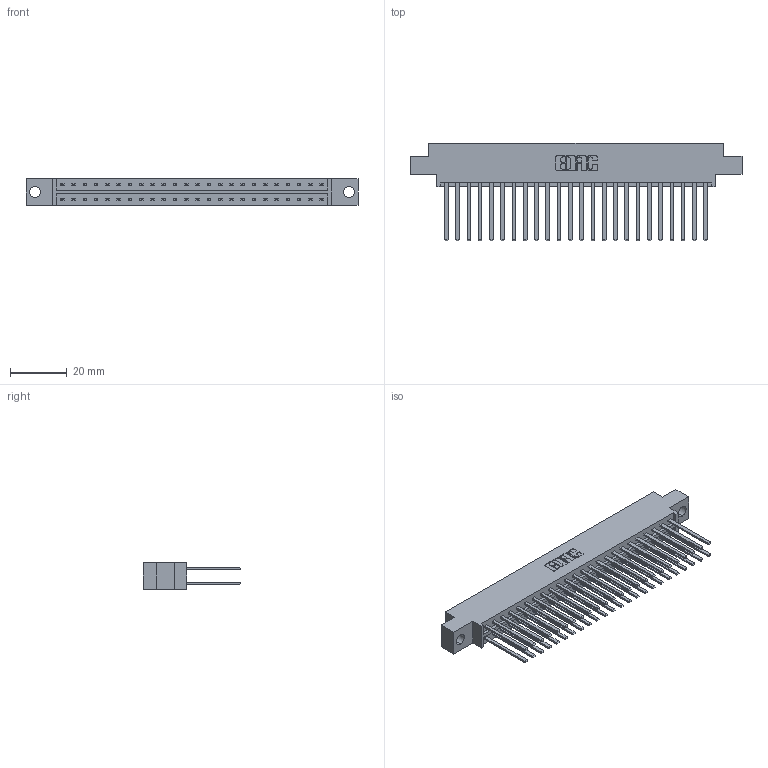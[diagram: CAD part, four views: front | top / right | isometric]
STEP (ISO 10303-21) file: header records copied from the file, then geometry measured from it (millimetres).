
FILE_DESCRIPTION (( 'STEP AP203' ), '1' );
FILE_NAME ('833-048-544-804.STEP', '2020-06-04T16:16:11', ( '' ), ( '' ), 'SwSTEP 2.0', 'SolidWorks 2020', '' );
FILE_SCHEMA (( 'CONFIG_CONTROL_DESIGN' ));
Length unit declared in the file: inch
Products named in the file (3): 833-048-544-804; 833 Part_Offset - .156 Dia - TH; 345-292-001_345-293-144
Assembly tree (49 placements, depth 2):
  833-048-544-804
    833 Part_Offset - .156 Dia - TH
    345-292-001_345-293-144  x48
Bounding box: 116.64 x 34.3 x 9.4 mm (x, y, z)
Volume: 12096.8 mm3; surface area: 16294.8 mm2
Topology: 49 solids, 49 shells, 2326 faces, 6899 edges, 4534 vertices
Faces by surface type: plane 1610, cylinder 716
Entity records: 17719 total; most frequent: CARTESIAN_POINT 2958, ORIENTED_EDGE 2894, DIRECTION 2555, EDGE_CURVE 1447, VECTOR 1323, LINE 1323, VERTEX_POINT 962, AXIS2_PLACEMENT_3D 616
